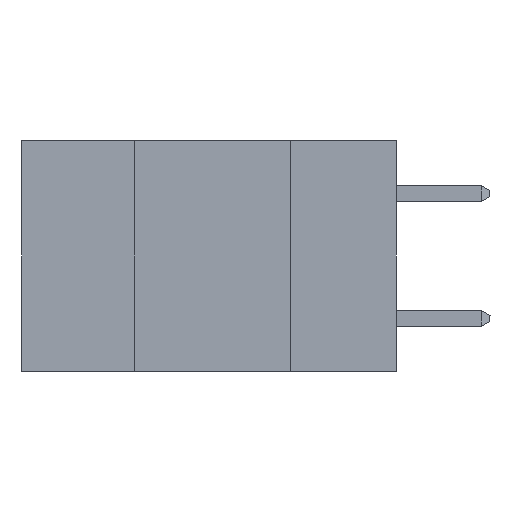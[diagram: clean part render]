
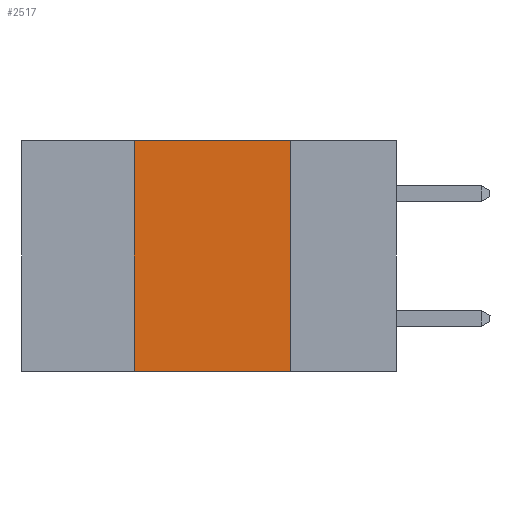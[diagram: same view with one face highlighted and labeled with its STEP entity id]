
A CAD part, left-side view. The second image highlights one B-rep face of the part: STEP entity #2517.
In plain terms, the highlighted planar face has unit normal (-1, 0, 0).
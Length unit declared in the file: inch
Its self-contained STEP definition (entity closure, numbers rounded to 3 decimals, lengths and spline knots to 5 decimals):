
#243 = EDGE_CURVE ( 'NONE', #9473, #11046, #6497, .T. ) ;
#244 = VECTOR ( 'NONE', #3488, 39.37008 ) ;
#748 = CARTESIAN_POINT ( 'NONE',  ( 0., 0.6, 0. ) ) ;
#1193 = EDGE_CURVE ( 'NONE', #9473, #8253, #7070, .T. ) ;
#1327 = CARTESIAN_POINT ( 'NONE',  ( 0., 0.42, -0.37 ) ) ;
#1441 = LINE ( 'NONE', #4175, #5493 ) ;
#1465 = DIRECTION ( 'NONE',  ( 0., 0., 1. ) ) ;
#2517 = ADVANCED_FACE ( 'NONE', ( #15047 ), #8243, .F. ) ;
#3076 = ORIENTED_EDGE ( 'NONE', *, *, #1193, .T. ) ;
#3488 = DIRECTION ( 'NONE',  ( 0., -1., 0. ) ) ;
#4175 = CARTESIAN_POINT ( 'NONE',  ( 0., 0.6, 0. ) ) ;
#4868 = DIRECTION ( 'NONE',  ( 0., 0., -1. ) ) ;
#5025 = DIRECTION ( 'NONE',  ( 1., 0., 0. ) ) ;
#5421 = EDGE_LOOP ( 'NONE', ( #14225, #7029, #10208, #3076 ) ) ;
#5493 = VECTOR ( 'NONE', #13548, 39.37008 ) ;
#5639 = CARTESIAN_POINT ( 'NONE',  ( 0., 0.17, -0.37 ) ) ;
#6497 = LINE ( 'NONE', #15907, #13239 ) ;
#7019 = CARTESIAN_POINT ( 'NONE',  ( 0., 0.17, -0.37 ) ) ;
#7029 = ORIENTED_EDGE ( 'NONE', *, *, #16295, .F. ) ;
#7056 = DIRECTION ( 'NONE',  ( 0., 0., -1. ) ) ;
#7070 = LINE ( 'NONE', #7151, #244 ) ;
#7151 = CARTESIAN_POINT ( 'NONE',  ( 0., 0.6, -0.37 ) ) ;
#7627 = LINE ( 'NONE', #7019, #13538 ) ;
#7846 = VERTEX_POINT ( 'NONE', #8522 ) ;
#8037 = EDGE_CURVE ( 'NONE', #7846, #8253, #7627, .T. ) ;
#8243 = PLANE ( 'NONE',  #14751 ) ;
#8253 = VERTEX_POINT ( 'NONE', #5639 ) ;
#8522 = CARTESIAN_POINT ( 'NONE',  ( 0., 0.17, 0. ) ) ;
#9473 = VERTEX_POINT ( 'NONE', #1327 ) ;
#9883 = CARTESIAN_POINT ( 'NONE',  ( 0., 0.42, 0. ) ) ;
#10208 = ORIENTED_EDGE ( 'NONE', *, *, #243, .F. ) ;
#11046 = VERTEX_POINT ( 'NONE', #9883 ) ;
#13239 = VECTOR ( 'NONE', #1465, 39.37008 ) ;
#13538 = VECTOR ( 'NONE', #7056, 39.37008 ) ;
#13548 = DIRECTION ( 'NONE',  ( 0., -1., 0. ) ) ;
#14225 = ORIENTED_EDGE ( 'NONE', *, *, #8037, .F. ) ;
#14751 = AXIS2_PLACEMENT_3D ( 'NONE', #748, #5025, #4868 ) ;
#15047 = FACE_OUTER_BOUND ( 'NONE', #5421, .T. ) ;
#15907 = CARTESIAN_POINT ( 'NONE',  ( 0., 0.42, -0.37 ) ) ;
#16295 = EDGE_CURVE ( 'NONE', #11046, #7846, #1441, .T. ) ;
